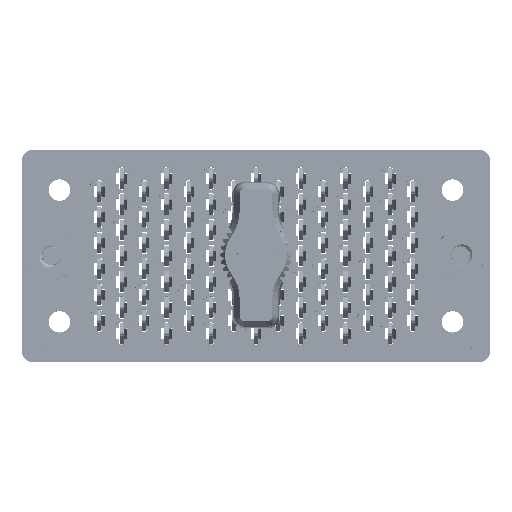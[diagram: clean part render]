
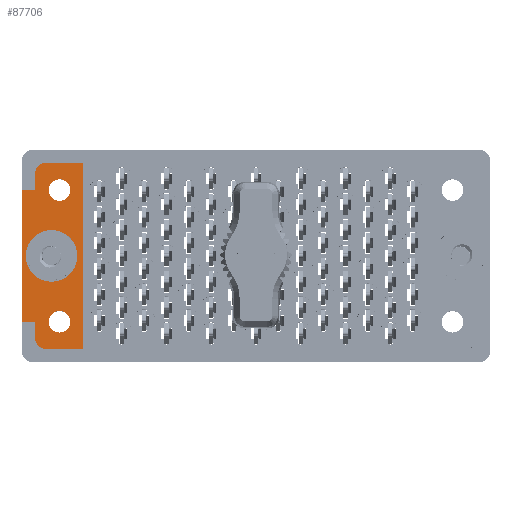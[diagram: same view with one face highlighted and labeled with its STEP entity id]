
A CAD part, top view. The second image highlights one B-rep face of the part: STEP entity #87706.
In plain terms, the highlighted planar face has unit normal (0, 0, 1).
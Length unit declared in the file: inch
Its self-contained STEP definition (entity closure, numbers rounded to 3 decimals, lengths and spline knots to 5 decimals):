
#452 = CARTESIAN_POINT ( 'NONE',  ( -1.359, -0.617, -0.117 ) ) ;
#1227 = VECTOR ( 'NONE', #42554, 39.37008 ) ;
#2922 = AXIS2_PLACEMENT_3D ( 'NONE', #79661, #18326, #87154 ) ;
#3805 = DIRECTION ( 'NONE',  ( 0., 0., 1. ) ) ;
#3859 = LINE ( 'NONE', #68565, #30702 ) ;
#4672 = CIRCLE ( 'NONE', #68846, 0.15 ) ;
#4834 = FACE_BOUND ( 'NONE', #52724, .T. ) ;
#5733 = CARTESIAN_POINT ( 'NONE',  ( -1.2825, -0.3825, -0.117 ) ) ;
#5737 = CARTESIAN_POINT ( 'NONE',  ( -1.2825, 0.478, -0.117 ) ) ;
#5806 = VERTEX_POINT ( 'NONE', #31565 ) ;
#6910 = CARTESIAN_POINT ( 'NONE',  ( 0., 0.3825, -0.117 ) ) ;
#7228 = EDGE_CURVE ( 'NONE', #95391, #23268, #30063, .T. ) ;
#8640 = VERTEX_POINT ( 'NONE', #9505 ) ;
#8717 = CARTESIAN_POINT ( 'NONE',  ( -1.3375, 0., -0.117 ) ) ;
#9505 = CARTESIAN_POINT ( 'NONE',  ( -1.2035, 0.3825, -0.117 ) ) ;
#9538 = VECTOR ( 'NONE', #46318, 39.37008 ) ;
#9639 = CARTESIAN_POINT ( 'NONE',  ( -1.2035, -0.3825, -0.117 ) ) ;
#9840 = EDGE_CURVE ( 'NONE', #17111, #88576, #93721, .T. ) ;
#10121 = DIRECTION ( 'NONE',  ( 1., 0., 0. ) ) ;
#10584 = CARTESIAN_POINT ( 'NONE',  ( -1.2205, 0.478, -0.117 ) ) ;
#10596 = FACE_OUTER_BOUND ( 'NONE', #77783, .T. ) ;
#12113 = VERTEX_POINT ( 'NONE', #50999 ) ;
#12248 = VERTEX_POINT ( 'NONE', #44143 ) ;
#12759 = CARTESIAN_POINT ( 'NONE',  ( -1.005, 0.617, -0.117 ) ) ;
#13074 = CARTESIAN_POINT ( 'NONE',  ( -1.141, 0.3825, -0.117 ) ) ;
#14973 = DIRECTION ( 'NONE',  ( 0., 0., 1. ) ) ;
#15444 = DIRECTION ( 'NONE',  ( 1., 0., 0. ) ) ;
#17111 = VERTEX_POINT ( 'NONE', #5733 ) ;
#17625 = FACE_BOUND ( 'NONE', #50229, .T. ) ;
#18326 = DIRECTION ( 'NONE',  ( 0., 0., 1. ) ) ;
#18523 = AXIS2_PLACEMENT_3D ( 'NONE', #452, #81988, #15444 ) ;
#18717 = VERTEX_POINT ( 'NONE', #67283 ) ;
#19085 = AXIS2_PLACEMENT_3D ( 'NONE', #71048, #3805, #85340 ) ;
#19753 = CARTESIAN_POINT ( 'NONE',  ( -1.2825, 0., -0.117 ) ) ;
#20028 = AXIS2_PLACEMENT_3D ( 'NONE', #68912, #91646, #24145 ) ;
#20082 = EDGE_CURVE ( 'NONE', #71601, #84385, #87977, .T. ) ;
#21809 = CARTESIAN_POINT ( 'NONE',  ( -1.359, 0.617, -0.117 ) ) ;
#23268 = VERTEX_POINT ( 'NONE', #5737 ) ;
#24145 = DIRECTION ( 'NONE',  ( 1., 0., 0. ) ) ;
#24616 = FACE_BOUND ( 'NONE', #71728, .T. ) ;
#25816 = DIRECTION ( 'NONE',  ( 0., 0., 1. ) ) ;
#26343 = EDGE_CURVE ( 'NONE', #31522, #88576, #42743, .T. ) ;
#27095 = CIRCLE ( 'NONE', #37232, 0.15 ) ;
#29064 = CARTESIAN_POINT ( 'NONE',  ( -1.359, 0.3825, -0.117 ) ) ;
#29527 = CARTESIAN_POINT ( 'NONE',  ( -1.0375, 0., -0.117 ) ) ;
#29611 = DIRECTION ( 'NONE',  ( -1., 0., 0. ) ) ;
#30063 = CIRCLE ( 'NONE', #82691, 0.062 ) ;
#30247 = ORIENTED_EDGE ( 'NONE', *, *, #72010, .F. ) ;
#30687 = EDGE_CURVE ( 'NONE', #17111, #12248, #3859, .T. ) ;
#30702 = VECTOR ( 'NONE', #82858, 39.37008 ) ;
#31522 = VERTEX_POINT ( 'NONE', #29064 ) ;
#31565 = CARTESIAN_POINT ( 'NONE',  ( -1.005, 0.54, -0.117 ) ) ;
#31732 = EDGE_CURVE ( 'NONE', #5806, #95391, #81870, .T. ) ;
#32992 = CARTESIAN_POINT ( 'NONE',  ( -1.1875, 0., -0.117 ) ) ;
#33872 = CARTESIAN_POINT ( 'NONE',  ( -1.2205, 0.54, -0.117 ) ) ;
#34544 = VERTEX_POINT ( 'NONE', #73635 ) ;
#35418 = ORIENTED_EDGE ( 'NONE', *, *, #89599, .T. ) ;
#36010 = EDGE_CURVE ( 'NONE', #55735, #56842, #27095, .T. ) ;
#37118 = VECTOR ( 'NONE', #58539, 39.37008 ) ;
#37177 = ORIENTED_EDGE ( 'NONE', *, *, #72341, .F. ) ;
#37216 = CIRCLE ( 'NONE', #19085, 0.062 ) ;
#37232 = AXIS2_PLACEMENT_3D ( 'NONE', #32992, #55596, #77998 ) ;
#39230 = VECTOR ( 'NONE', #67214, 39.37008 ) ;
#39979 = EDGE_CURVE ( 'NONE', #82595, #31522, #87223, .T. ) ;
#42554 = DIRECTION ( 'NONE',  ( 0., 1., 0. ) ) ;
#42637 = LINE ( 'NONE', #19753, #44966 ) ;
#42743 = LINE ( 'NONE', #21809, #39230 ) ;
#44143 = CARTESIAN_POINT ( 'NONE',  ( -1.2825, -0.478, -0.117 ) ) ;
#44966 = VECTOR ( 'NONE', #57703, 39.37008 ) ;
#45028 = CARTESIAN_POINT ( 'NONE',  ( 0., 0.54, -0.117 ) ) ;
#45142 = CARTESIAN_POINT ( 'NONE',  ( -1.359, -0.3825, -0.117 ) ) ;
#45554 = ORIENTED_EDGE ( 'NONE', *, *, #39979, .T. ) ;
#46318 = DIRECTION ( 'NONE',  ( -1., 0., 0. ) ) ;
#46813 = LINE ( 'NONE', #12759, #1227 ) ;
#48112 = CARTESIAN_POINT ( 'NONE',  ( -1.141, -0.3825, -0.117 ) ) ;
#48367 = CIRCLE ( 'NONE', #20028, 0.0625 ) ;
#48754 = DIRECTION ( 'NONE',  ( 1., 0., 0. ) ) ;
#48894 = ORIENTED_EDGE ( 'NONE', *, *, #50526, .T. ) ;
#49818 = ORIENTED_EDGE ( 'NONE', *, *, #20082, .F. ) ;
#50229 = EDGE_LOOP ( 'NONE', ( #37177, #70923 ) ) ;
#50526 = EDGE_CURVE ( 'NONE', #34544, #5806, #46813, .T. ) ;
#50999 = CARTESIAN_POINT ( 'NONE',  ( -1.0785, 0.3825, -0.117 ) ) ;
#51933 = EDGE_CURVE ( 'NONE', #84385, #71601, #48367, .T. ) ;
#52724 = EDGE_LOOP ( 'NONE', ( #30247, #96147 ) ) ;
#53374 = CARTESIAN_POINT ( 'NONE',  ( 0., -0.3825, -0.117 ) ) ;
#55596 = DIRECTION ( 'NONE',  ( 0., 0., 1. ) ) ;
#55610 = ORIENTED_EDGE ( 'NONE', *, *, #26343, .T. ) ;
#55735 = VERTEX_POINT ( 'NONE', #8717 ) ;
#56842 = VERTEX_POINT ( 'NONE', #29527 ) ;
#57703 = DIRECTION ( 'NONE',  ( 0., -1., 0. ) ) ;
#57974 = DIRECTION ( 'NONE',  ( 1., 0., 0. ) ) ;
#58539 = DIRECTION ( 'NONE',  ( -1., 0., 0. ) ) ;
#60382 = ORIENTED_EDGE ( 'NONE', *, *, #30687, .T. ) ;
#60790 = CIRCLE ( 'NONE', #80096, 0.0625 ) ;
#61522 = CARTESIAN_POINT ( 'NONE',  ( -1.0785, -0.3825, -0.117 ) ) ;
#61846 = LINE ( 'NONE', #91313, #95606 ) ;
#62853 = CIRCLE ( 'NONE', #2922, 0.0625 ) ;
#65481 = ORIENTED_EDGE ( 'NONE', *, *, #51933, .F. ) ;
#65755 = ORIENTED_EDGE ( 'NONE', *, *, #69148, .T. ) ;
#67102 = ORIENTED_EDGE ( 'NONE', *, *, #88799, .F. ) ;
#67214 = DIRECTION ( 'NONE',  ( 0., -1., 0. ) ) ;
#67283 = CARTESIAN_POINT ( 'NONE',  ( -1.2205, -0.54, -0.117 ) ) ;
#68565 = CARTESIAN_POINT ( 'NONE',  ( -1.2825, 0., -0.117 ) ) ;
#68846 = AXIS2_PLACEMENT_3D ( 'NONE', #69546, #92608, #10121 ) ;
#68912 = CARTESIAN_POINT ( 'NONE',  ( -1.141, -0.3825, -0.117 ) ) ;
#69148 = EDGE_CURVE ( 'NONE', #23268, #82595, #42637, .T. ) ;
#69546 = CARTESIAN_POINT ( 'NONE',  ( -1.1875, 0., -0.117 ) ) ;
#70511 = DIRECTION ( 'NONE',  ( -1., 0., 0. ) ) ;
#70613 = CARTESIAN_POINT ( 'NONE',  ( -1.2825, 0.3825, -0.117 ) ) ;
#70923 = ORIENTED_EDGE ( 'NONE', *, *, #36010, .F. ) ;
#71048 = CARTESIAN_POINT ( 'NONE',  ( -1.2205, -0.478, -0.117 ) ) ;
#71601 = VERTEX_POINT ( 'NONE', #61522 ) ;
#71728 = EDGE_LOOP ( 'NONE', ( #65481, #49818 ) ) ;
#72010 = EDGE_CURVE ( 'NONE', #8640, #12113, #60790, .T. ) ;
#72341 = EDGE_CURVE ( 'NONE', #56842, #55735, #4672, .T. ) ;
#73635 = CARTESIAN_POINT ( 'NONE',  ( -1.005, -0.54, -0.117 ) ) ;
#73915 = VECTOR ( 'NONE', #29611, 39.37008 ) ;
#77783 = EDGE_LOOP ( 'NONE', ( #60382, #35418, #67102, #48894, #90646, #91718, #65755, #45554, #55610, #93522 ) ) ;
#77998 = DIRECTION ( 'NONE',  ( 1., 0., 0. ) ) ;
#78836 = EDGE_CURVE ( 'NONE', #12113, #8640, #62853, .T. ) ;
#79661 = CARTESIAN_POINT ( 'NONE',  ( -1.141, 0.3825, -0.117 ) ) ;
#80096 = AXIS2_PLACEMENT_3D ( 'NONE', #13074, #89040, #95559 ) ;
#81870 = LINE ( 'NONE', #45028, #9538 ) ;
#81988 = DIRECTION ( 'NONE',  ( 0., 0., 1. ) ) ;
#82267 = AXIS2_PLACEMENT_3D ( 'NONE', #48112, #25816, #48754 ) ;
#82595 = VERTEX_POINT ( 'NONE', #70613 ) ;
#82691 = AXIS2_PLACEMENT_3D ( 'NONE', #10584, #14973, #57974 ) ;
#82858 = DIRECTION ( 'NONE',  ( 0., -1., 0. ) ) ;
#84385 = VERTEX_POINT ( 'NONE', #9639 ) ;
#85340 = DIRECTION ( 'NONE',  ( 1., 0., 0. ) ) ;
#87154 = DIRECTION ( 'NONE',  ( 1., 0., 0. ) ) ;
#87223 = LINE ( 'NONE', #6910, #37118 ) ;
#87706 = ADVANCED_FACE ( 'NONE', ( #24616, #4834, #17625, #10596 ), #90767, .T. ) ;
#87977 = CIRCLE ( 'NONE', #82267, 0.0625 ) ;
#88576 = VERTEX_POINT ( 'NONE', #45142 ) ;
#88799 = EDGE_CURVE ( 'NONE', #34544, #18717, #61846, .T. ) ;
#89040 = DIRECTION ( 'NONE',  ( 0., 0., 1. ) ) ;
#89599 = EDGE_CURVE ( 'NONE', #12248, #18717, #37216, .T. ) ;
#90646 = ORIENTED_EDGE ( 'NONE', *, *, #31732, .T. ) ;
#90767 = PLANE ( 'NONE',  #18523 ) ;
#91313 = CARTESIAN_POINT ( 'NONE',  ( 0., -0.54, -0.117 ) ) ;
#91646 = DIRECTION ( 'NONE',  ( 0., 0., 1. ) ) ;
#91718 = ORIENTED_EDGE ( 'NONE', *, *, #7228, .T. ) ;
#92608 = DIRECTION ( 'NONE',  ( 0., 0., 1. ) ) ;
#93522 = ORIENTED_EDGE ( 'NONE', *, *, #9840, .F. ) ;
#93721 = LINE ( 'NONE', #53374, #73915 ) ;
#95391 = VERTEX_POINT ( 'NONE', #33872 ) ;
#95559 = DIRECTION ( 'NONE',  ( 1., 0., 0. ) ) ;
#95606 = VECTOR ( 'NONE', #70511, 39.37008 ) ;
#96147 = ORIENTED_EDGE ( 'NONE', *, *, #78836, .F. ) ;
